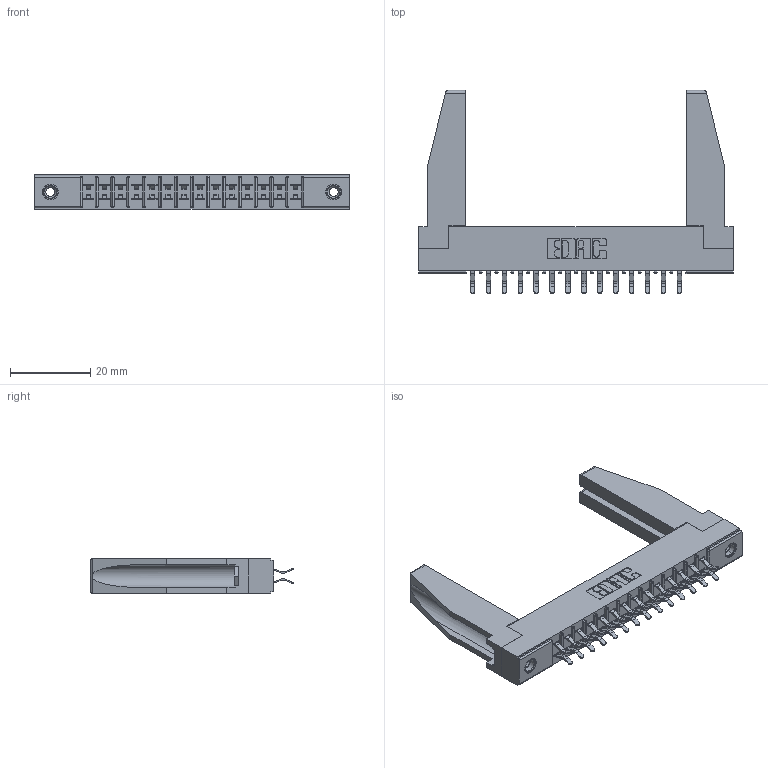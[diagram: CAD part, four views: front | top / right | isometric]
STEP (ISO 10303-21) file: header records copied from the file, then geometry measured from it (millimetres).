
FILE_DESCRIPTION (( 'STEP AP203' ), '1' );
FILE_NAME ('315-028-556-278.STEP', '2019-09-10T15:16:43', ( '' ), ( '' ), 'SwSTEP 2.0', 'SolidWorks 2016', '' );
FILE_SCHEMA (( 'CONFIG_CONTROL_DESIGN' ));
Length unit declared in the file: inch
Products named in the file (5): 305 Part_.156 Dia; 345-250-001_345-250-001-102; 305-290-001_556; 307-220-078; 315-028-556-278
Assembly tree (33 placements, depth 2):
  315-028-556-278
    305 Part_.156 Dia
    305-290-001_556  x28
    345-250-001_345-250-001-102  x2
    307-220-078  x2
Bounding box: 78.49 x 50.67 x 8.71 mm (x, y, z)
Volume: 8927.7 mm3; surface area: 12670.9 mm2
Topology: 33 solids, 33 shells, 1814 faces, 5168 edges, 3360 vertices
Faces by surface type: plane 1020, cylinder 722, sphere 56, cone 12, torus 4
Entity records: 21228 total; most frequent: CARTESIAN_POINT 3522, ORIENTED_EDGE 3450, DIRECTION 3391, EDGE_CURVE 1725, VECTOR 1357, LINE 1357, VERTEX_POINT 1106, AXIS2_PLACEMENT_3D 1017
